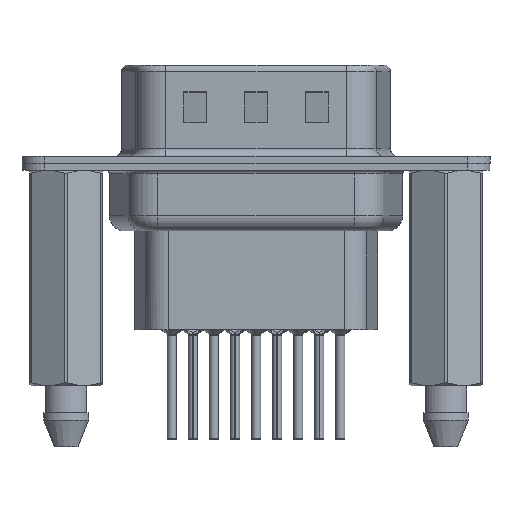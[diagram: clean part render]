
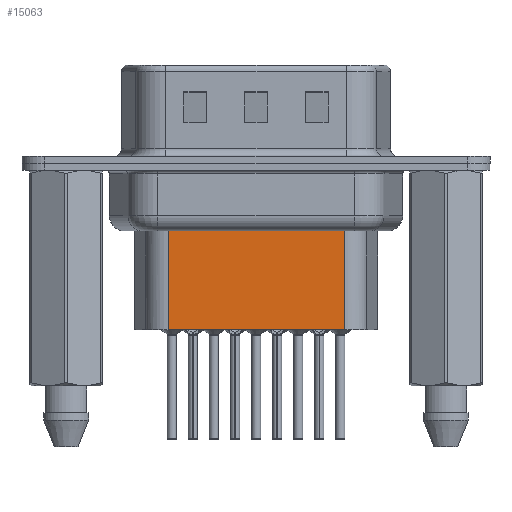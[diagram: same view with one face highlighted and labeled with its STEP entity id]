
A CAD part, front view. The second image highlights one B-rep face of the part: STEP entity #15063.
In plain terms, the highlighted planar face has unit normal (0, -1, 0).
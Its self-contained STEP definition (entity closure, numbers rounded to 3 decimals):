
#267 = AXIS2_PLACEMENT_3D ( 'NONE', #4880, #14472, #17714 ) ;
#268 = ORIENTED_EDGE ( 'NONE', *, *, #4920, .F. ) ;
#283 = CARTESIAN_POINT ( 'NONE',  ( 18.294, -3.5, -3.1 ) ) ;
#979 = LINE ( 'NONE', #10571, #7146 ) ;
#2404 = ORIENTED_EDGE ( 'NONE', *, *, #16395, .F. ) ;
#3520 = ORIENTED_EDGE ( 'NONE', *, *, #20473, .T. ) ;
#4278 = VECTOR ( 'NONE', #6015, 1000. ) ;
#4880 = CARTESIAN_POINT ( 'NONE',  ( 6.706, -3.5, -3.1 ) ) ;
#4920 = EDGE_CURVE ( 'NONE', #10188, #12100, #979, .T. ) ;
#5547 = ORIENTED_EDGE ( 'NONE', *, *, #9850, .T. ) ;
#5798 = VECTOR ( 'NONE', #11901, 1000. ) ;
#6015 = DIRECTION ( 'NONE',  ( -1., 0., 0. ) ) ;
#6510 = LINE ( 'NONE', #13070, #11394 ) ;
#7146 = VECTOR ( 'NONE', #14102, 1000. ) ;
#7816 = DIRECTION ( 'NONE',  ( 0., 0., -1. ) ) ;
#9850 = EDGE_CURVE ( 'NONE', #15452, #17931, #12291, .T. ) ;
#10188 = VERTEX_POINT ( 'NONE', #13554 ) ;
#10319 = CARTESIAN_POINT ( 'NONE',  ( 6.706, -3.5, -10.95 ) ) ;
#10571 = CARTESIAN_POINT ( 'NONE',  ( 6.706, -3.5, -10.95 ) ) ;
#11394 = VECTOR ( 'NONE', #7816, 1000. ) ;
#11901 = DIRECTION ( 'NONE',  ( 0., 0., -1. ) ) ;
#12010 = LINE ( 'NONE', #283, #5798 ) ;
#12100 = VERTEX_POINT ( 'NONE', #10319 ) ;
#12291 = LINE ( 'NONE', #15608, #4278 ) ;
#13070 = CARTESIAN_POINT ( 'NONE',  ( 6.706, -3.5, -3.1 ) ) ;
#13554 = CARTESIAN_POINT ( 'NONE',  ( 18.294, -3.5, -10.95 ) ) ;
#14102 = DIRECTION ( 'NONE',  ( -1., 0., 0. ) ) ;
#14472 = DIRECTION ( 'NONE',  ( 0., -1., 0. ) ) ;
#15063 = ADVANCED_FACE ( 'NONE', ( #21277 ), #19444, .T. ) ;
#15452 = VERTEX_POINT ( 'NONE', #16486 ) ;
#15608 = CARTESIAN_POINT ( 'NONE',  ( 6.459, -3.5, -4.097 ) ) ;
#16395 = EDGE_CURVE ( 'NONE', #15452, #10188, #12010, .T. ) ;
#16486 = CARTESIAN_POINT ( 'NONE',  ( 18.294, -3.5, -4.097 ) ) ;
#17714 = DIRECTION ( 'NONE',  ( 1., 0., 0. ) ) ;
#17931 = VERTEX_POINT ( 'NONE', #20387 ) ;
#19257 = EDGE_LOOP ( 'NONE', ( #2404, #5547, #3520, #268 ) ) ;
#19444 = PLANE ( 'NONE',  #267 ) ;
#20387 = CARTESIAN_POINT ( 'NONE',  ( 6.706, -3.5, -4.097 ) ) ;
#20473 = EDGE_CURVE ( 'NONE', #17931, #12100, #6510, .T. ) ;
#21277 = FACE_OUTER_BOUND ( 'NONE', #19257, .T. ) ;
